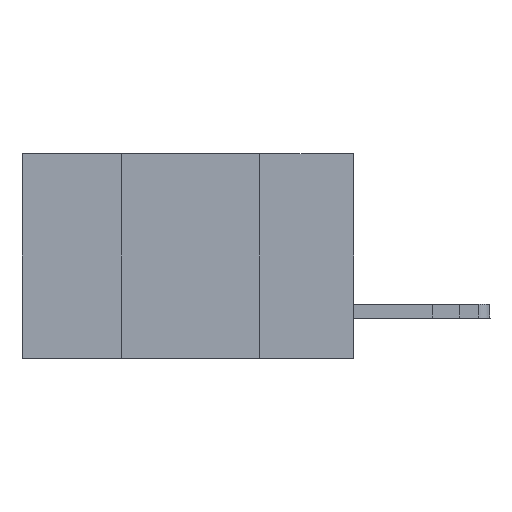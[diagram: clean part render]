
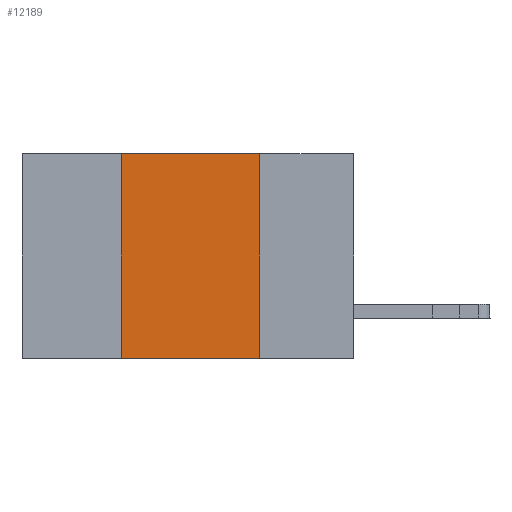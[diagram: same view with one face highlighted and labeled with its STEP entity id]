
A CAD part, left-side view. The second image highlights one B-rep face of the part: STEP entity #12189.
In plain terms, the highlighted planar face has unit normal (-1, 0, 0).
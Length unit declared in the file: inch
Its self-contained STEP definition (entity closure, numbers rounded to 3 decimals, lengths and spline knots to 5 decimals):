
#1027 = LINE ( 'NONE', #20602, #4889 ) ;
#1103 = CARTESIAN_POINT ( 'NONE',  ( 0., 0.17, 0. ) ) ;
#1646 = EDGE_CURVE ( 'NONE', #10618, #4552, #7567, .T. ) ;
#2094 = AXIS2_PLACEMENT_3D ( 'NONE', #5640, #14046, #15373 ) ;
#3155 = EDGE_CURVE ( 'NONE', #5135, #4552, #16103, .T. ) ;
#3653 = VECTOR ( 'NONE', #6477, 39.37008 ) ;
#3807 = ORIENTED_EDGE ( 'NONE', *, *, #1646, .F. ) ;
#4552 = VERTEX_POINT ( 'NONE', #13793 ) ;
#4889 = VECTOR ( 'NONE', #12724, 39.37008 ) ;
#5135 = VERTEX_POINT ( 'NONE', #20106 ) ;
#5640 = CARTESIAN_POINT ( 'NONE',  ( 0., 0.6, 0. ) ) ;
#5958 = CARTESIAN_POINT ( 'NONE',  ( 0., 0.17, 0. ) ) ;
#6393 = DIRECTION ( 'NONE',  ( 0., 0., 1. ) ) ;
#6477 = DIRECTION ( 'NONE',  ( 0., -1., 0. ) ) ;
#7455 = FACE_OUTER_BOUND ( 'NONE', #18378, .T. ) ;
#7567 = LINE ( 'NONE', #5958, #13816 ) ;
#9152 = PLANE ( 'NONE',  #2094 ) ;
#10618 = VERTEX_POINT ( 'NONE', #1103 ) ;
#10887 = LINE ( 'NONE', #21060, #14808 ) ;
#11481 = CARTESIAN_POINT ( 'NONE',  ( 0., 0.42, 0. ) ) ;
#11644 = ORIENTED_EDGE ( 'NONE', *, *, #14651, .F. ) ;
#12189 = ADVANCED_FACE ( 'NONE', ( #7455 ), #9152, .F. ) ;
#12724 = DIRECTION ( 'NONE',  ( 0., -1., 0. ) ) ;
#13793 = CARTESIAN_POINT ( 'NONE',  ( 0., 0.17, -0.37 ) ) ;
#13816 = VECTOR ( 'NONE', #16114, 39.37008 ) ;
#14046 = DIRECTION ( 'NONE',  ( 1., 0., 0. ) ) ;
#14254 = EDGE_CURVE ( 'NONE', #5135, #21018, #10887, .T. ) ;
#14651 = EDGE_CURVE ( 'NONE', #21018, #10618, #1027, .T. ) ;
#14808 = VECTOR ( 'NONE', #6393, 39.37008 ) ;
#15110 = ORIENTED_EDGE ( 'NONE', *, *, #14254, .F. ) ;
#15373 = DIRECTION ( 'NONE',  ( 0., 0., -1. ) ) ;
#16103 = LINE ( 'NONE', #21162, #3653 ) ;
#16114 = DIRECTION ( 'NONE',  ( 0., 0., -1. ) ) ;
#18161 = ORIENTED_EDGE ( 'NONE', *, *, #3155, .T. ) ;
#18378 = EDGE_LOOP ( 'NONE', ( #3807, #11644, #15110, #18161 ) ) ;
#20106 = CARTESIAN_POINT ( 'NONE',  ( 0., 0.42, -0.37 ) ) ;
#20602 = CARTESIAN_POINT ( 'NONE',  ( 0., 0.6, 0. ) ) ;
#21018 = VERTEX_POINT ( 'NONE', #11481 ) ;
#21060 = CARTESIAN_POINT ( 'NONE',  ( 0., 0.42, 0. ) ) ;
#21162 = CARTESIAN_POINT ( 'NONE',  ( 0., 0.6, -0.37 ) ) ;
